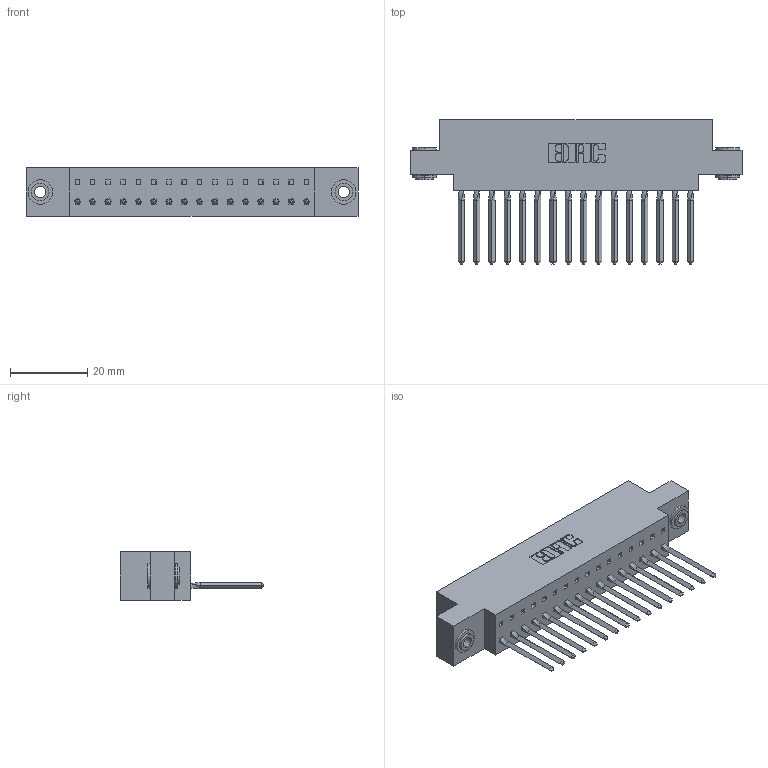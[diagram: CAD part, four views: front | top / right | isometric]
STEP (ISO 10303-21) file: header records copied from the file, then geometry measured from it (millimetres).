
FILE_DESCRIPTION (( 'STEP AP203' ), '1' );
FILE_NAME ('317-016-541-603.STEP', '2020-02-27T15:14:51', ( '' ), ( '' ), 'SwSTEP 2.0', 'SolidWorks 2016', '' );
FILE_SCHEMA (( 'CONFIG_CONTROL_DESIGN' ));
Length unit declared in the file: inch
Products named in the file (4): 317-016-541-603; 317 Part_.156 Dia - TH; 317-290-002_541; 345-250-002_345-250-002-102
Assembly tree (19 placements, depth 2):
  317-016-541-603
    317 Part_.156 Dia - TH
    317-290-002_541  x16
    345-250-002_345-250-002-102  x2
Bounding box: 86.11 x 37.34 x 12.7 mm (x, y, z)
Volume: 13183.4 mm3; surface area: 17976.9 mm2
Topology: 19 solids, 19 shells, 2572 faces, 7295 edges, 4742 vertices
Faces by surface type: plane 2052, cylinder 448, bspline 64, cone 8
Entity records: 28441 total; most frequent: CARTESIAN_POINT 5652, ORIENTED_EDGE 4914, DIRECTION 4059, EDGE_CURVE 2457, LINE 2069, VECTOR 2069, VERTEX_POINT 1628, AXIS2_PLACEMENT_3D 995
